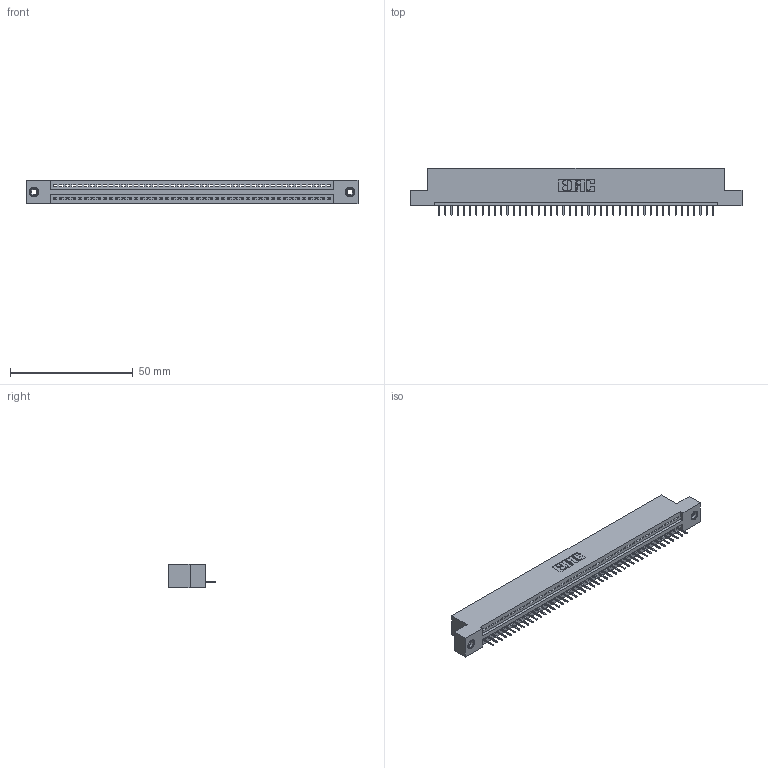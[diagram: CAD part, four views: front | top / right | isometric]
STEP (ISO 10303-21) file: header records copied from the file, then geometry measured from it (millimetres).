
FILE_DESCRIPTION (( 'STEP AP203' ), '1' );
FILE_NAME ('395-045-524-108.STEP', '2019-10-22T18:17:11', ( '' ), ( '' ), 'SwSTEP 2.0', 'SolidWorks 2016', '' );
FILE_SCHEMA (( 'CONFIG_CONTROL_DESIGN' ));
Length unit declared in the file: inch
Products named in the file (4): 395-045-524-108; 345-292-001_345-293-124; 345-250-001_345-250-003-102; 345 Part_Flush Mounting Lugs - 0.156 Dia-TI
Assembly tree (48 placements, depth 2):
  395-045-524-108
    345 Part_Flush Mounting Lugs - 0.156 Dia-TI
    345-292-001_345-293-124  x45
    345-250-001_345-250-003-102  x2
Bounding box: 135.51 x 19.35 x 9.4 mm (x, y, z)
Volume: 12711.1 mm3; surface area: 16383.4 mm2
Topology: 48 solids, 48 shells, 2976 faces, 8577 edges, 5530 vertices
Faces by surface type: plane 2182, cylinder 778, cone 12, torus 4
Entity records: 34724 total; most frequent: CARTESIAN_POINT 5994, ORIENTED_EDGE 5966, DIRECTION 5259, EDGE_CURVE 2983, LINE 2655, VECTOR 2655, VERTEX_POINT 1980, AXIS2_PLACEMENT_3D 1302
